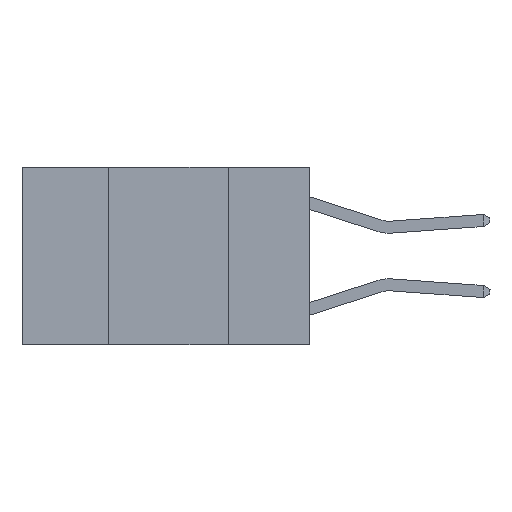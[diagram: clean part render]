
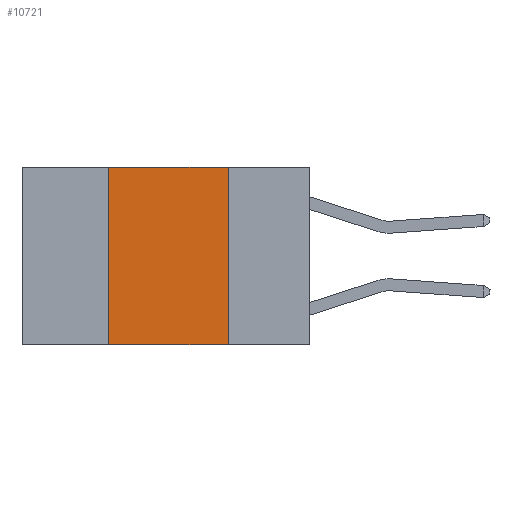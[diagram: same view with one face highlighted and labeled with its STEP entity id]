
A CAD part, left-side view. The second image highlights one B-rep face of the part: STEP entity #10721.
In plain terms, the highlighted planar face has unit normal (-1, 0, 0).
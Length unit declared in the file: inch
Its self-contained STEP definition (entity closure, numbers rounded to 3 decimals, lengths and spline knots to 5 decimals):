
#12 = LINE ( 'NONE', #18390, #8152 ) ;
#319 = EDGE_CURVE ( 'NONE', #5626, #8401, #20186, .T. ) ;
#775 = CARTESIAN_POINT ( 'NONE',  ( 0., 0.42, 0. ) ) ;
#1137 = AXIS2_PLACEMENT_3D ( 'NONE', #15198, #5390, #16831 ) ;
#1244 = ORIENTED_EDGE ( 'NONE', *, *, #9055, .F. ) ;
#3764 = PLANE ( 'NONE',  #1137 ) ;
#3776 = VECTOR ( 'NONE', #17451, 39.37008 ) ;
#4687 = EDGE_CURVE ( 'NONE', #5626, #4727, #12107, .T. ) ;
#4727 = VERTEX_POINT ( 'NONE', #775 ) ;
#5238 = CARTESIAN_POINT ( 'NONE',  ( 0., 0.6, -0.37 ) ) ;
#5390 = DIRECTION ( 'NONE',  ( 1., 0., 0. ) ) ;
#5529 = CARTESIAN_POINT ( 'NONE',  ( 0., 0.42, 0. ) ) ;
#5626 = VERTEX_POINT ( 'NONE', #17418 ) ;
#6033 = CARTESIAN_POINT ( 'NONE',  ( 0., 0.17, 0. ) ) ;
#8152 = VECTOR ( 'NONE', #8611, 39.37008 ) ;
#8401 = VERTEX_POINT ( 'NONE', #9781 ) ;
#8611 = DIRECTION ( 'NONE',  ( 0., -1., 0. ) ) ;
#9055 = EDGE_CURVE ( 'NONE', #11993, #8401, #20097, .T. ) ;
#9563 = FACE_OUTER_BOUND ( 'NONE', #15502, .T. ) ;
#9781 = CARTESIAN_POINT ( 'NONE',  ( 0., 0.17, -0.37 ) ) ;
#10188 = CARTESIAN_POINT ( 'NONE',  ( 0., 0.17, 0. ) ) ;
#10721 = ADVANCED_FACE ( 'NONE', ( #9563 ), #3764, .F. ) ;
#10740 = ORIENTED_EDGE ( 'NONE', *, *, #12001, .F. ) ;
#11993 = VERTEX_POINT ( 'NONE', #10188 ) ;
#12001 = EDGE_CURVE ( 'NONE', #4727, #11993, #12, .T. ) ;
#12107 = LINE ( 'NONE', #5529, #20269 ) ;
#12278 = ORIENTED_EDGE ( 'NONE', *, *, #4687, .F. ) ;
#15198 = CARTESIAN_POINT ( 'NONE',  ( 0., 0.6, 0. ) ) ;
#15502 = EDGE_LOOP ( 'NONE', ( #1244, #10740, #12278, #19531 ) ) ;
#16831 = DIRECTION ( 'NONE',  ( 0., 0., -1. ) ) ;
#17418 = CARTESIAN_POINT ( 'NONE',  ( 0., 0.42, -0.37 ) ) ;
#17451 = DIRECTION ( 'NONE',  ( 0., 0., -1. ) ) ;
#18356 = DIRECTION ( 'NONE',  ( 0., -1., 0. ) ) ;
#18390 = CARTESIAN_POINT ( 'NONE',  ( 0., 0.6, 0. ) ) ;
#18583 = DIRECTION ( 'NONE',  ( 0., 0., 1. ) ) ;
#19531 = ORIENTED_EDGE ( 'NONE', *, *, #319, .T. ) ;
#19678 = VECTOR ( 'NONE', #18356, 39.37008 ) ;
#20097 = LINE ( 'NONE', #6033, #3776 ) ;
#20186 = LINE ( 'NONE', #5238, #19678 ) ;
#20269 = VECTOR ( 'NONE', #18583, 39.37008 ) ;
